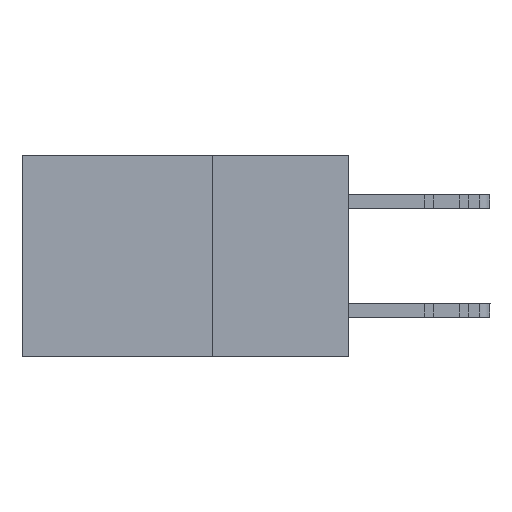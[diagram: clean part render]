
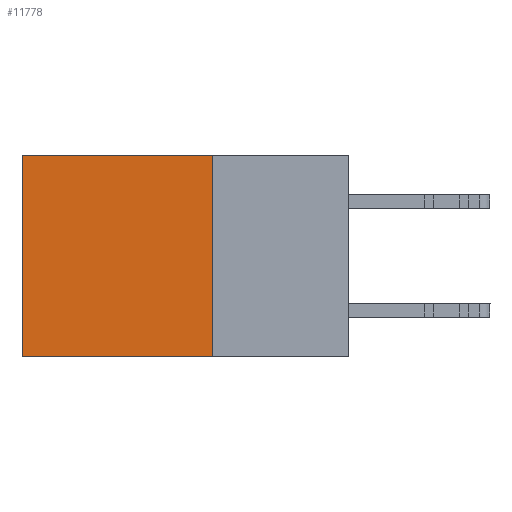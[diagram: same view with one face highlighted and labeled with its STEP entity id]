
A CAD part, left-side view. The second image highlights one B-rep face of the part: STEP entity #11778.
In plain terms, the highlighted planar face has unit normal (-1, 0, 0).
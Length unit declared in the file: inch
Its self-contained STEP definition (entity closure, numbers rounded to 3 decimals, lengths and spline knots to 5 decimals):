
#1557 = VECTOR ( 'NONE', #16496, 39.37008 ) ;
#2605 = ORIENTED_EDGE ( 'NONE', *, *, #9701, .T. ) ;
#3132 = DIRECTION ( 'NONE',  ( 0., 1., 0. ) ) ;
#4839 = PLANE ( 'NONE',  #13787 ) ;
#5028 = DIRECTION ( 'NONE',  ( 0., 0., -1. ) ) ;
#5465 = ORIENTED_EDGE ( 'NONE', *, *, #17551, .F. ) ;
#5585 = CARTESIAN_POINT ( 'NONE',  ( 0.298, 0.25, 0. ) ) ;
#6027 = DIRECTION ( 'NONE',  ( 0., 0., -1. ) ) ;
#6811 = CARTESIAN_POINT ( 'NONE',  ( 0.298, 0.25, 0. ) ) ;
#7194 = EDGE_LOOP ( 'NONE', ( #23191, #5465, #11868, #2605 ) ) ;
#7540 = VECTOR ( 'NONE', #14092, 39.37008 ) ;
#8909 = LINE ( 'NONE', #5585, #1557 ) ;
#9022 = FACE_OUTER_BOUND ( 'NONE', #7194, .T. ) ;
#9701 = EDGE_CURVE ( 'NONE', #10947, #24838, #8909, .T. ) ;
#10947 = VERTEX_POINT ( 'NONE', #6811 ) ;
#11778 = ADVANCED_FACE ( 'NONE', ( #9022 ), #4839, .F. ) ;
#11868 = ORIENTED_EDGE ( 'NONE', *, *, #14956, .F. ) ;
#13787 = AXIS2_PLACEMENT_3D ( 'NONE', #24973, #22784, #5028 ) ;
#14092 = DIRECTION ( 'NONE',  ( 0., 0., -1. ) ) ;
#14956 = EDGE_CURVE ( 'NONE', #10947, #25977, #22545, .T. ) ;
#16496 = DIRECTION ( 'NONE',  ( 0., 1., 0. ) ) ;
#16604 = CARTESIAN_POINT ( 'NONE',  ( 0.298, 0.25, -0.37 ) ) ;
#17148 = CARTESIAN_POINT ( 'NONE',  ( 0.298, 0.25, -0.37 ) ) ;
#17551 = EDGE_CURVE ( 'NONE', #25977, #25948, #24830, .T. ) ;
#18795 = CARTESIAN_POINT ( 'NONE',  ( 0.298, 0.6, -0.37 ) ) ;
#19470 = LINE ( 'NONE', #25274, #7540 ) ;
#19819 = CARTESIAN_POINT ( 'NONE',  ( 0.298, 0.25, 0. ) ) ;
#19957 = CARTESIAN_POINT ( 'NONE',  ( 0.298, 0.6, 0. ) ) ;
#22008 = VECTOR ( 'NONE', #3132, 39.37008 ) ;
#22545 = LINE ( 'NONE', #19819, #24326 ) ;
#22784 = DIRECTION ( 'NONE',  ( 1., 0., 0. ) ) ;
#23191 = ORIENTED_EDGE ( 'NONE', *, *, #28836, .T. ) ;
#24326 = VECTOR ( 'NONE', #6027, 39.37008 ) ;
#24830 = LINE ( 'NONE', #16604, #22008 ) ;
#24838 = VERTEX_POINT ( 'NONE', #19957 ) ;
#24973 = CARTESIAN_POINT ( 'NONE',  ( 0.298, 0.25, 0. ) ) ;
#25274 = CARTESIAN_POINT ( 'NONE',  ( 0.298, 0.6, 0. ) ) ;
#25948 = VERTEX_POINT ( 'NONE', #18795 ) ;
#25977 = VERTEX_POINT ( 'NONE', #17148 ) ;
#28836 = EDGE_CURVE ( 'NONE', #24838, #25948, #19470, .T. ) ;
